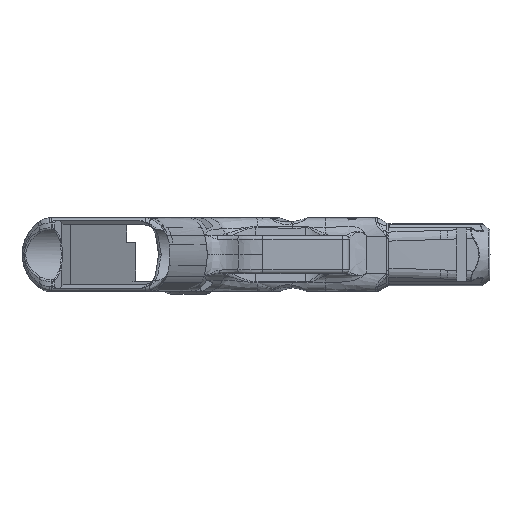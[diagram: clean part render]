
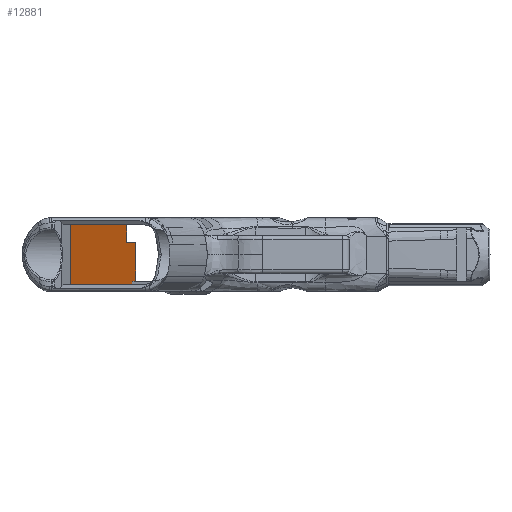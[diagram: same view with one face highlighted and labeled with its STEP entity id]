
A CAD part, front view. The second image highlights one B-rep face of the part: STEP entity #12881.
In plain terms, the highlighted planar face has unit normal (0.951, -0.309, 0).
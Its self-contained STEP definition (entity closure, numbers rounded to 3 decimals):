
#556=PLANE('',#13849);
#1983=FACE_OUTER_BOUND('',#2663,.T.);
#2663=EDGE_LOOP('',(#12039,#12040,#12041,#12042,#12043,#12044,#12045,#12046));
#3350=LINE('',#24735,#4034);
#3446=LINE('',#27173,#4130);
#3464=LINE('',#28329,#4148);
#3517=LINE('',#36661,#4201);
#3531=LINE('',#36849,#4215);
#3552=LINE('',#38920,#4236);
#3553=LINE('',#38986,#4237);
#3562=LINE('',#39486,#4246);
#4034=VECTOR('',#14720,10.);
#4130=VECTOR('',#14990,10.);
#4148=VECTOR('',#15088,10.);
#4201=VECTOR('',#15371,10.);
#4215=VECTOR('',#15391,10.);
#4236=VECTOR('',#15474,10.);
#4237=VECTOR('',#15481,10.);
#4246=VECTOR('',#15532,10.);
#5542=VERTEX_POINT('',#24733);
#5543=VERTEX_POINT('',#24734);
#5714=VERTEX_POINT('',#27170);
#5715=VERTEX_POINT('',#27172);
#5921=VERTEX_POINT('',#36660);
#5930=VERTEX_POINT('',#36814);
#5934=VERTEX_POINT('',#36847);
#5979=VERTEX_POINT('',#38985);
#6942=EDGE_CURVE('',#5542,#5543,#3350,.T.);
#7166=EDGE_CURVE('',#5715,#5714,#3446,.T.);
#7244=EDGE_CURVE('',#5542,#5714,#3464,.T.);
#7501=EDGE_CURVE('',#5715,#5921,#3517,.T.);
#7521=EDGE_CURVE('',#5934,#5930,#3531,.T.);
#7587=EDGE_CURVE('',#5921,#5934,#3552,.T.);
#7590=EDGE_CURVE('',#5930,#5979,#3553,.T.);
#7619=EDGE_CURVE('',#5979,#5543,#3562,.T.);
#12039=ORIENTED_EDGE('',*,*,#7244,.F.);
#12040=ORIENTED_EDGE('',*,*,#6942,.T.);
#12041=ORIENTED_EDGE('',*,*,#7619,.F.);
#12042=ORIENTED_EDGE('',*,*,#7590,.F.);
#12043=ORIENTED_EDGE('',*,*,#7521,.F.);
#12044=ORIENTED_EDGE('',*,*,#7587,.F.);
#12045=ORIENTED_EDGE('',*,*,#7501,.F.);
#12046=ORIENTED_EDGE('',*,*,#7166,.T.);
#12881=ADVANCED_FACE('',(#1983),#556,.F.);
#13849=AXIS2_PLACEMENT_3D('',#53875,#16405,#16406);
#14720=DIRECTION('',(0.309,0.951,0.));
#14990=DIRECTION('',(-0.309,-0.951,0.));
#15088=DIRECTION('',(0.,0.,1.));
#15371=DIRECTION('',(0.,0.,-1.));
#15391=DIRECTION('',(0.,0.,-1.));
#15474=DIRECTION('',(0.309,0.951,0.));
#15481=DIRECTION('',(-0.309,-0.951,0.));
#15532=DIRECTION('',(0.,0.,-1.));
#16405=DIRECTION('center_axis',(-0.951,0.309,0.));
#16406=DIRECTION('ref_axis',(0.,0.,
1.));
#24733=CARTESIAN_POINT('',(8.112,-79.915,-11.75));
#24734=CARTESIAN_POINT('',(32.169,-5.875,-11.75));
#24735=CARTESIAN_POINT('',(2.312,-97.765,-11.75));
#27170=CARTESIAN_POINT('',(8.112,-79.915,11.75));
#27172=CARTESIAN_POINT('',(30.049,-12.4,11.75));
#27173=CARTESIAN_POINT('',(2.312,-97.765,11.75));
#28329=CARTESIAN_POINT('',(8.112,-79.915,-13.075));
#36660=CARTESIAN_POINT('',(30.049,-12.4,4.75));
#36661=CARTESIAN_POINT('',(30.049,-12.4,2.982));
#36814=CARTESIAN_POINT('',(33.591,-1.5,-10.375));
#36847=CARTESIAN_POINT('',(33.591,-1.5,4.75));
#36849=CARTESIAN_POINT('',(33.591,-1.5,-5.875));
#38920=CARTESIAN_POINT('',(18.86,-46.836,4.75));
#38985=CARTESIAN_POINT('',(32.169,-5.875,-10.375));
#38986=CARTESIAN_POINT('',(17.241,-51.82,-10.375));
#39486=CARTESIAN_POINT('',(32.169,-5.875,-5.875));
#53875=CARTESIAN_POINT('Origin',(2.312,-97.765,-11.75));
